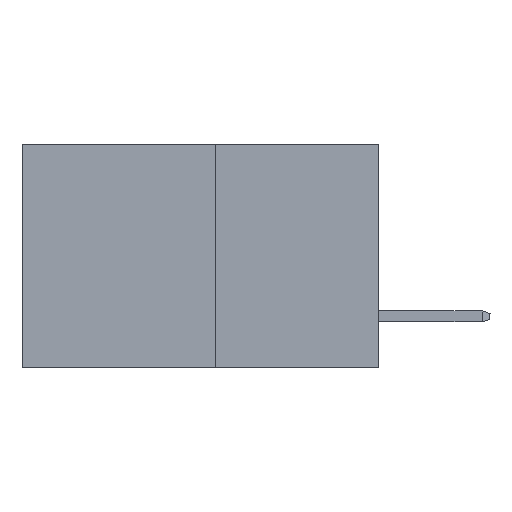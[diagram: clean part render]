
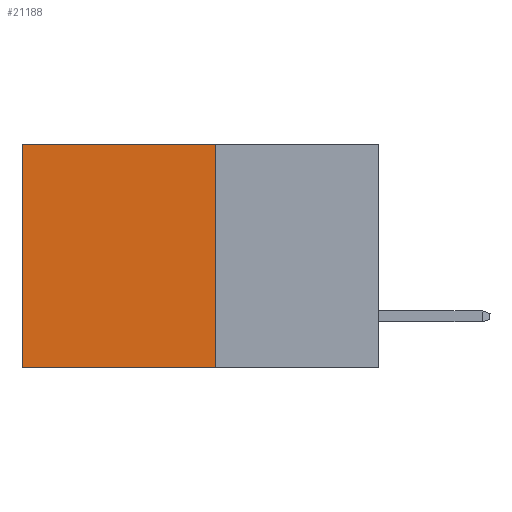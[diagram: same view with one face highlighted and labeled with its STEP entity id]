
A CAD part, left-side view. The second image highlights one B-rep face of the part: STEP entity #21188.
In plain terms, the highlighted planar face has unit normal (-1, 0, 0).
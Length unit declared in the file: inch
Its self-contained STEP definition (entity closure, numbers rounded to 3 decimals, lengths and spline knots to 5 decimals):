
#276 = CARTESIAN_POINT ( 'NONE',  ( 0.277, 0.27, -0.37 ) ) ;
#1670 = VECTOR ( 'NONE', #21855, 39.37008 ) ;
#1943 = VERTEX_POINT ( 'NONE', #18069 ) ;
#3817 = CARTESIAN_POINT ( 'NONE',  ( 0.277, 0.27, -0.37 ) ) ;
#4814 = ORIENTED_EDGE ( 'NONE', *, *, #10625, .T. ) ;
#5627 = AXIS2_PLACEMENT_3D ( 'NONE', #3817, #24420, #12050 ) ;
#6384 = VERTEX_POINT ( 'NONE', #16401 ) ;
#6634 = CARTESIAN_POINT ( 'NONE',  ( 0.277, 0.27, 0. ) ) ;
#6671 = EDGE_CURVE ( 'NONE', #6384, #17348, #24586, .T. ) ;
#6961 = ORIENTED_EDGE ( 'NONE', *, *, #22780, .F. ) ;
#8650 = VECTOR ( 'NONE', #17155, 39.37008 ) ;
#8658 = DIRECTION ( 'NONE',  ( 0., 1., 0. ) ) ;
#9493 = CARTESIAN_POINT ( 'NONE',  ( 0.277, 0.27, -0.37 ) ) ;
#9892 = CARTESIAN_POINT ( 'NONE',  ( 0.277, 0.59, -0.37 ) ) ;
#9974 = DIRECTION ( 'NONE',  ( 0., 0., -1. ) ) ;
#10625 = EDGE_CURVE ( 'NONE', #1943, #6384, #17071, .T. ) ;
#10635 = ORIENTED_EDGE ( 'NONE', *, *, #6671, .T. ) ;
#12050 = DIRECTION ( 'NONE',  ( 0., 0., -1. ) ) ;
#12556 = FACE_OUTER_BOUND ( 'NONE', #24901, .T. ) ;
#13262 = LINE ( 'NONE', #9493, #1670 ) ;
#15779 = VERTEX_POINT ( 'NONE', #276 ) ;
#16306 = ORIENTED_EDGE ( 'NONE', *, *, #16929, .F. ) ;
#16401 = CARTESIAN_POINT ( 'NONE',  ( 0.277, 0.59, 0. ) ) ;
#16929 = EDGE_CURVE ( 'NONE', #15779, #17348, #13262, .T. ) ;
#17071 = LINE ( 'NONE', #6634, #21928 ) ;
#17155 = DIRECTION ( 'NONE',  ( 0., 0., -1. ) ) ;
#17348 = VERTEX_POINT ( 'NONE', #23263 ) ;
#18069 = CARTESIAN_POINT ( 'NONE',  ( 0.277, 0.27, 0. ) ) ;
#21188 = ADVANCED_FACE ( 'NONE', ( #12556 ), #22374, .F. ) ;
#21855 = DIRECTION ( 'NONE',  ( 0., 1., 0. ) ) ;
#21928 = VECTOR ( 'NONE', #8658, 39.37008 ) ;
#22374 = PLANE ( 'NONE',  #5627 ) ;
#22780 = EDGE_CURVE ( 'NONE', #1943, #15779, #25070, .T. ) ;
#23263 = CARTESIAN_POINT ( 'NONE',  ( 0.277, 0.59, -0.37 ) ) ;
#23943 = VECTOR ( 'NONE', #9974, 39.37008 ) ;
#24420 = DIRECTION ( 'NONE',  ( 1., 0., 0. ) ) ;
#24586 = LINE ( 'NONE', #9892, #23943 ) ;
#24901 = EDGE_LOOP ( 'NONE', ( #10635, #16306, #6961, #4814 ) ) ;
#25070 = LINE ( 'NONE', #25331, #8650 ) ;
#25331 = CARTESIAN_POINT ( 'NONE',  ( 0.277, 0.27, -0.37 ) ) ;
